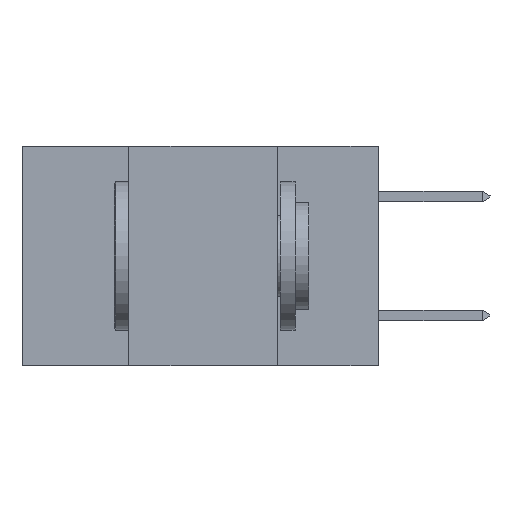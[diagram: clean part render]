
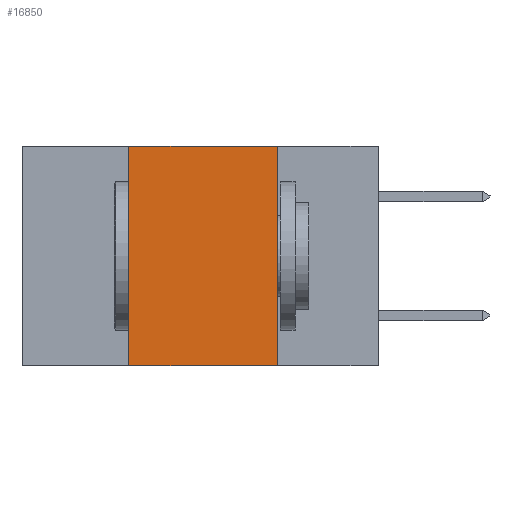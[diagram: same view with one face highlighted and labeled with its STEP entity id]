
A CAD part, left-side view. The second image highlights one B-rep face of the part: STEP entity #16850.
In plain terms, the highlighted planar face has unit normal (-1, 0, 0).
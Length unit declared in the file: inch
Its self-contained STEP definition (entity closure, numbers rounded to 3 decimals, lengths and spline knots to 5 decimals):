
#756 = LINE ( 'NONE', #17496, #7514 ) ;
#964 = EDGE_CURVE ( 'NONE', #7954, #13647, #9830, .T. ) ;
#1015 = DIRECTION ( 'NONE',  ( 0., 0., 1. ) ) ;
#1275 = VECTOR ( 'NONE', #8633, 39.37008 ) ;
#2390 = VERTEX_POINT ( 'NONE', #3349 ) ;
#2664 = LINE ( 'NONE', #5326, #3524 ) ;
#3043 = CARTESIAN_POINT ( 'NONE',  ( 0., 0.17, -0.37 ) ) ;
#3349 = CARTESIAN_POINT ( 'NONE',  ( 0., 0.42, 0. ) ) ;
#3524 = VECTOR ( 'NONE', #1015, 39.37008 ) ;
#3632 = DIRECTION ( 'NONE',  ( 0., 0., -1. ) ) ;
#4219 = EDGE_CURVE ( 'NONE', #2390, #15275, #756, .T. ) ;
#5191 = FACE_OUTER_BOUND ( 'NONE', #11247, .T. ) ;
#5264 = ORIENTED_EDGE ( 'NONE', *, *, #964, .T. ) ;
#5326 = CARTESIAN_POINT ( 'NONE',  ( 0., 0.42, -0.37 ) ) ;
#5742 = DIRECTION ( 'NONE',  ( 0., 0., -1. ) ) ;
#6149 = CARTESIAN_POINT ( 'NONE',  ( 0., 0.42, -0.37 ) ) ;
#7477 = EDGE_CURVE ( 'NONE', #15275, #13647, #15489, .T. ) ;
#7514 = VECTOR ( 'NONE', #7637, 39.37008 ) ;
#7637 = DIRECTION ( 'NONE',  ( 0., -1., 0. ) ) ;
#7954 = VERTEX_POINT ( 'NONE', #6149 ) ;
#8633 = DIRECTION ( 'NONE',  ( 0., -1., 0. ) ) ;
#9018 = ORIENTED_EDGE ( 'NONE', *, *, #4219, .F. ) ;
#9183 = VECTOR ( 'NONE', #5742, 39.37008 ) ;
#9830 = LINE ( 'NONE', #11471, #1275 ) ;
#10991 = DIRECTION ( 'NONE',  ( 1., 0., 0. ) ) ;
#11247 = EDGE_LOOP ( 'NONE', ( #13230, #9018, #17067, #5264 ) ) ;
#11471 = CARTESIAN_POINT ( 'NONE',  ( 0., 0.6, -0.37 ) ) ;
#12719 = CARTESIAN_POINT ( 'NONE',  ( 0., 0.17, -0.37 ) ) ;
#13230 = ORIENTED_EDGE ( 'NONE', *, *, #7477, .F. ) ;
#13464 = PLANE ( 'NONE',  #17320 ) ;
#13647 = VERTEX_POINT ( 'NONE', #3043 ) ;
#14560 = EDGE_CURVE ( 'NONE', #7954, #2390, #2664, .T. ) ;
#15275 = VERTEX_POINT ( 'NONE', #15595 ) ;
#15489 = LINE ( 'NONE', #12719, #9183 ) ;
#15595 = CARTESIAN_POINT ( 'NONE',  ( 0., 0.17, 0. ) ) ;
#16404 = CARTESIAN_POINT ( 'NONE',  ( 0., 0.6, 0. ) ) ;
#16850 = ADVANCED_FACE ( 'NONE', ( #5191 ), #13464, .F. ) ;
#17067 = ORIENTED_EDGE ( 'NONE', *, *, #14560, .F. ) ;
#17320 = AXIS2_PLACEMENT_3D ( 'NONE', #16404, #10991, #3632 ) ;
#17496 = CARTESIAN_POINT ( 'NONE',  ( 0., 0.6, 0. ) ) ;
